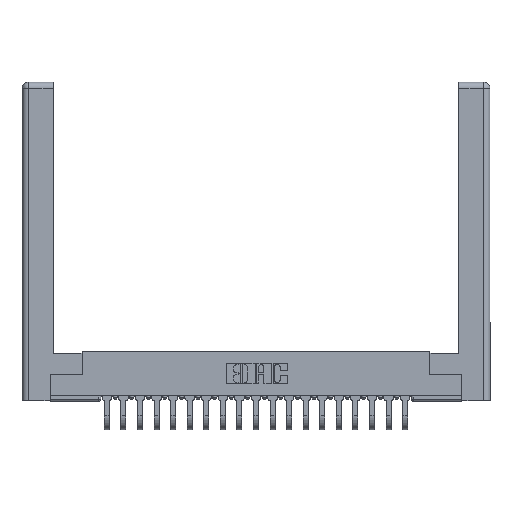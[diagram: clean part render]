
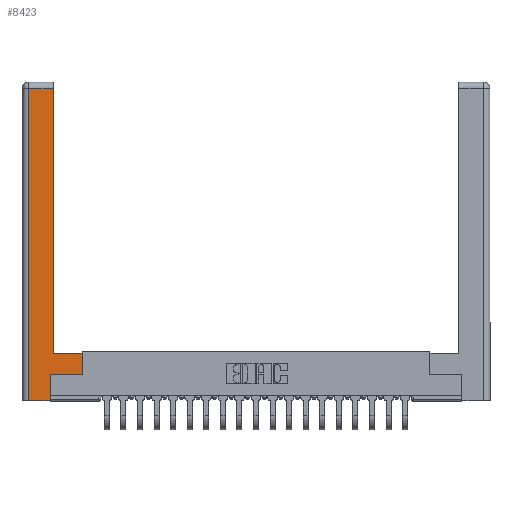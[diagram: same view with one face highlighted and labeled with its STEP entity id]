
A CAD part, top view. The second image highlights one B-rep face of the part: STEP entity #8423.
In plain terms, the highlighted planar face has unit normal (0, 0, 1).
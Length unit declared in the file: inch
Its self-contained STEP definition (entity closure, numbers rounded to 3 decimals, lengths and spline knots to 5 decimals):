
#85 = VECTOR ( 'NONE', #15592, 39.37008 ) ;
#578 = CARTESIAN_POINT ( 'NONE',  ( 0.295, 3., 0. ) ) ;
#643 = VECTOR ( 'NONE', #1593, 39.37008 ) ;
#767 = CARTESIAN_POINT ( 'NONE',  ( 0.295, 0.45, 0. ) ) ;
#976 = CARTESIAN_POINT ( 'NONE',  ( 0.265, 0., 0. ) ) ;
#1336 = LINE ( 'NONE', #21461, #19013 ) ;
#1431 = VECTOR ( 'NONE', #4471, 39.37008 ) ;
#1448 = ORIENTED_EDGE ( 'NONE', *, *, #15098, .T. ) ;
#1593 = DIRECTION ( 'NONE',  ( 1., 0., 0. ) ) ;
#1976 = CARTESIAN_POINT ( 'NONE',  ( 0.265, 0., 0. ) ) ;
#2253 = ORIENTED_EDGE ( 'NONE', *, *, #21450, .T. ) ;
#2339 = ORIENTED_EDGE ( 'NONE', *, *, #12561, .T. ) ;
#2767 = DIRECTION ( 'NONE',  ( -1., 0., 0. ) ) ;
#2999 = ORIENTED_EDGE ( 'NONE', *, *, #3908, .T. ) ;
#3139 = CARTESIAN_POINT ( 'NONE',  ( 0.565, 0.45, 0. ) ) ;
#3421 = DIRECTION ( 'NONE',  ( 0., 1., 0. ) ) ;
#3908 = EDGE_CURVE ( 'NONE', #13546, #17495, #16925, .T. ) ;
#3985 = VERTEX_POINT ( 'NONE', #7472 ) ;
#4361 = CARTESIAN_POINT ( 'NONE',  ( 0.0615, 0., 0. ) ) ;
#4471 = DIRECTION ( 'NONE',  ( -1., 0., 0. ) ) ;
#4603 = CARTESIAN_POINT ( 'NONE',  ( 0., 0., 0. ) ) ;
#4761 = VECTOR ( 'NONE', #3421, 39.37008 ) ;
#5320 = CARTESIAN_POINT ( 'NONE',  ( 0.0615, 2.94, 0. ) ) ;
#5911 = DIRECTION ( 'NONE',  ( 0., -1., 0. ) ) ;
#6615 = VERTEX_POINT ( 'NONE', #767 ) ;
#7301 = DIRECTION ( 'NONE',  ( 0., 1., 0. ) ) ;
#7472 = CARTESIAN_POINT ( 'NONE',  ( 0.565, 0.45, 0. ) ) ;
#8423 = ADVANCED_FACE ( 'NONE', ( #9915 ), #10023, .F. ) ;
#8720 = LINE ( 'NONE', #1976, #85 ) ;
#9474 = ORIENTED_EDGE ( 'NONE', *, *, #17461, .T. ) ;
#9878 = DIRECTION ( 'NONE',  ( 0., 1., 0. ) ) ;
#9915 = FACE_OUTER_BOUND ( 'NONE', #12686, .T. ) ;
#10023 = PLANE ( 'NONE',  #18902 ) ;
#10109 = LINE ( 'NONE', #21840, #643 ) ;
#10469 = CARTESIAN_POINT ( 'NONE',  ( 0.265, 0.245, 0. ) ) ;
#10945 = VECTOR ( 'NONE', #7301, 39.37008 ) ;
#11023 = EDGE_CURVE ( 'NONE', #17495, #12177, #10109, .T. ) ;
#11044 = VERTEX_POINT ( 'NONE', #5320 ) ;
#12177 = VERTEX_POINT ( 'NONE', #17680 ) ;
#12561 = EDGE_CURVE ( 'NONE', #3985, #6615, #19641, .T. ) ;
#12686 = EDGE_LOOP ( 'NONE', ( #2253, #21364, #1448, #9474, #2999, #15441, #20293, #2339 ) ) ;
#12825 = VERTEX_POINT ( 'NONE', #13646 ) ;
#12900 = DIRECTION ( 'NONE',  ( -1., 0., 0. ) ) ;
#12955 = CARTESIAN_POINT ( 'NONE',  ( 0.295, 2.94, 0. ) ) ;
#13238 = DIRECTION ( 'NONE',  ( 0., 0., -1. ) ) ;
#13546 = VERTEX_POINT ( 'NONE', #976 ) ;
#13646 = CARTESIAN_POINT ( 'NONE',  ( 0.0615, 0., 0. ) ) ;
#14045 = VECTOR ( 'NONE', #5911, 39.37008 ) ;
#15098 = EDGE_CURVE ( 'NONE', #11044, #12825, #17876, .T. ) ;
#15441 = ORIENTED_EDGE ( 'NONE', *, *, #11023, .T. ) ;
#15592 = DIRECTION ( 'NONE',  ( 1., 0., 0. ) ) ;
#16118 = CARTESIAN_POINT ( 'NONE',  ( 0.295, 0.45, 0. ) ) ;
#16169 = EDGE_CURVE ( 'NONE', #21585, #11044, #1336, .T. ) ;
#16925 = LINE ( 'NONE', #21671, #4761 ) ;
#17015 = EDGE_CURVE ( 'NONE', #12177, #3985, #21828, .T. ) ;
#17401 = LINE ( 'NONE', #578, #10945 ) ;
#17461 = EDGE_CURVE ( 'NONE', #12825, #13546, #8720, .T. ) ;
#17495 = VERTEX_POINT ( 'NONE', #10469 ) ;
#17680 = CARTESIAN_POINT ( 'NONE',  ( 0.565, 0.245, 0. ) ) ;
#17876 = LINE ( 'NONE', #4361, #14045 ) ;
#17902 = VECTOR ( 'NONE', #9878, 39.37008 ) ;
#18902 = AXIS2_PLACEMENT_3D ( 'NONE', #4603, #13238, #12900 ) ;
#19013 = VECTOR ( 'NONE', #2767, 39.37008 ) ;
#19641 = LINE ( 'NONE', #16118, #1431 ) ;
#20293 = ORIENTED_EDGE ( 'NONE', *, *, #17015, .T. ) ;
#21364 = ORIENTED_EDGE ( 'NONE', *, *, #16169, .T. ) ;
#21450 = EDGE_CURVE ( 'NONE', #6615, #21585, #17401, .T. ) ;
#21461 = CARTESIAN_POINT ( 'NONE',  ( 0.0615, 2.94, 0. ) ) ;
#21585 = VERTEX_POINT ( 'NONE', #12955 ) ;
#21671 = CARTESIAN_POINT ( 'NONE',  ( 0.265, 0.245, 0. ) ) ;
#21828 = LINE ( 'NONE', #3139, #17902 ) ;
#21840 = CARTESIAN_POINT ( 'NONE',  ( 0.565, 0.245, 0. ) ) ;
